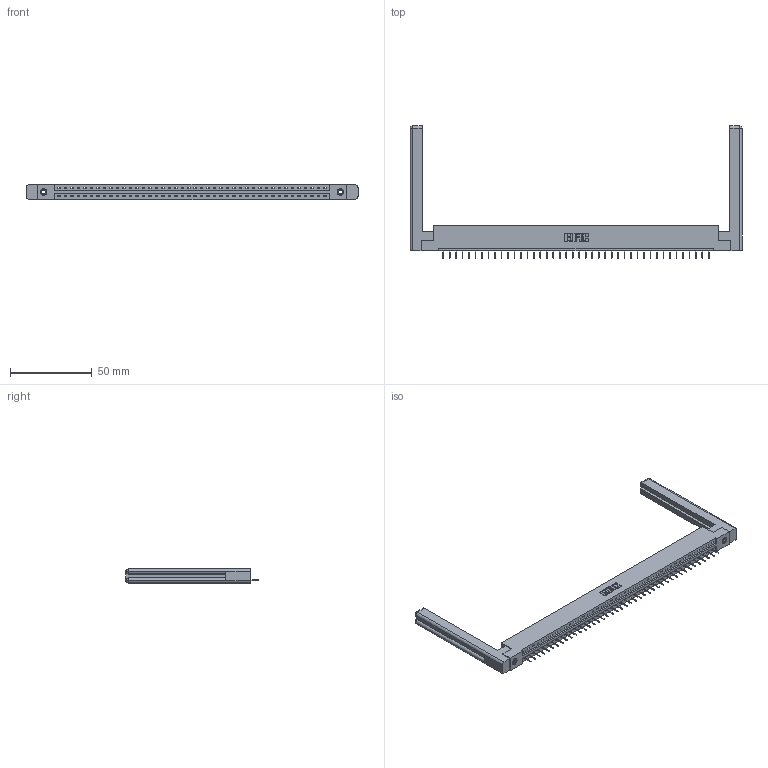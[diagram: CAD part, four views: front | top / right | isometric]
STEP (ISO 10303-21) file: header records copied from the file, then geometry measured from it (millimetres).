
FILE_DESCRIPTION (( 'STEP AP203' ), '1' );
FILE_NAME ('387-042-524-158.STEP', '2019-10-04T20:50:14', ( '' ), ( '' ), 'SwSTEP 2.0', 'SolidWorks 2016', '' );
FILE_SCHEMA (( 'CONFIG_CONTROL_DESIGN' ));
Length unit declared in the file: inch
Products named in the file (5): 307-220-058; 387-042-524-158; 345-250-001_345-250-001-102; 345-292-001_345-293-124; 337 Part_Flush Mounting Lugs - 0.156 Dia-TI
Assembly tree (47 placements, depth 2):
  387-042-524-158
    337 Part_Flush Mounting Lugs - 0.156 Dia-TI
    345-292-001_345-293-124  x42
    345-250-001_345-250-001-102  x2
    307-220-058  x2
Bounding box: 203.05 x 80.78 x 9.4 mm (x, y, z)
Volume: 28099.6 mm3; surface area: 26265.4 mm2
Topology: 47 solids, 47 shells, 3028 faces, 8729 edges, 5638 vertices
Faces by surface type: plane 2338, cylinder 666, cone 12, torus 12
Entity records: 33928 total; most frequent: CARTESIAN_POINT 5907, ORIENTED_EDGE 5824, DIRECTION 4992, EDGE_CURVE 2912, VECTOR 2740, LINE 2740, VERTEX_POINT 1930, AXIS2_PLACEMENT_3D 1126
